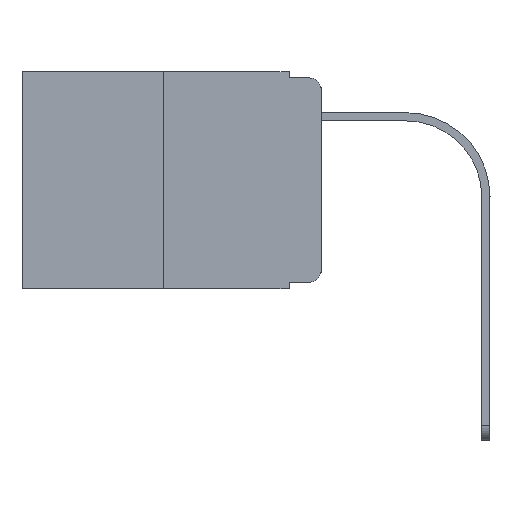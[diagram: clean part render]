
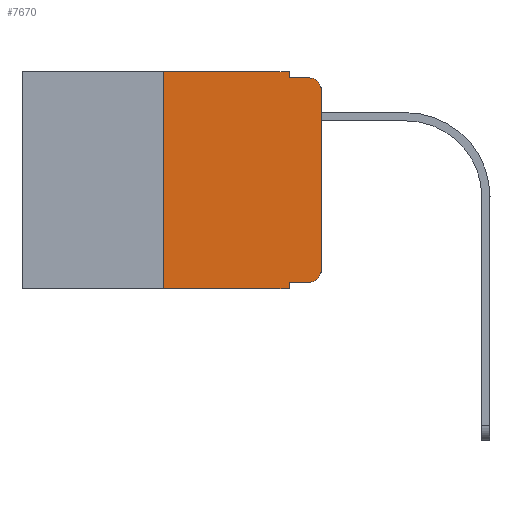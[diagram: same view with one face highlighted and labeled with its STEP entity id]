
A CAD part, left-side view. The second image highlights one B-rep face of the part: STEP entity #7670.
In plain terms, the highlighted planar face has unit normal (-1, 0, 0).
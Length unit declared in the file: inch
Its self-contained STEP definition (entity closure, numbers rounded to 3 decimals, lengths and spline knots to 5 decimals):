
#72 = ORIENTED_EDGE ( 'NONE', *, *, #3887, .T. ) ;
#78 = DIRECTION ( 'NONE',  ( -1., 0., 0. ) ) ;
#151 = CARTESIAN_POINT ( 'NONE',  ( 0., 0.473, 0. ) ) ;
#175 = VERTEX_POINT ( 'NONE', #3811 ) ;
#650 = CARTESIAN_POINT ( 'NONE',  ( 0., 0.25, 0. ) ) ;
#834 = FACE_OUTER_BOUND ( 'NONE', #10438, .T. ) ;
#1130 = VECTOR ( 'NONE', #8430, 39.37008 ) ;
#1160 = DIRECTION ( 'NONE',  ( 0., 0., -1. ) ) ;
#1174 = LINE ( 'NONE', #5401, #1667 ) ;
#1454 = VERTEX_POINT ( 'NONE', #7032 ) ;
#1511 = LINE ( 'NONE', #5705, #4065 ) ;
#1522 = EDGE_CURVE ( 'NONE', #1454, #3395, #8868, .T. ) ;
#1667 = VECTOR ( 'NONE', #9541, 39.37008 ) ;
#1795 = DIRECTION ( 'NONE',  ( 0., -1., 0. ) ) ;
#1896 = DIRECTION ( 'NONE',  ( 1., 0., 0. ) ) ;
#1957 = LINE ( 'NONE', #151, #4524 ) ;
#2030 = VERTEX_POINT ( 'NONE', #5943 ) ;
#2083 = CARTESIAN_POINT ( 'NONE',  ( 0., 0.051, -0.333 ) ) ;
#2164 = CARTESIAN_POINT ( 'NONE',  ( 0., 0., 0. ) ) ;
#2345 = CARTESIAN_POINT ( 'NONE',  ( 0., 0., -0.313 ) ) ;
#2362 = VERTEX_POINT ( 'NONE', #10074 ) ;
#2467 = EDGE_CURVE ( 'NONE', #8702, #10439, #1957, .T. ) ;
#2486 = CARTESIAN_POINT ( 'NONE',  ( 0., 0.051, 0. ) ) ;
#2540 = EDGE_CURVE ( 'NONE', #6546, #175, #1174, .T. ) ;
#2632 = LINE ( 'NONE', #6116, #4465 ) ;
#2684 = DIRECTION ( 'NONE',  ( 0., 0., -1. ) ) ;
#2714 = CARTESIAN_POINT ( 'NONE',  ( 0., 0., -0.03 ) ) ;
#2738 = EDGE_CURVE ( 'NONE', #3395, #8111, #6498, .T. ) ;
#2785 = EDGE_CURVE ( 'NONE', #6546, #8702, #4998, .T. ) ;
#2924 = LINE ( 'NONE', #2083, #3303 ) ;
#3303 = VECTOR ( 'NONE', #3873, 39.37008 ) ;
#3395 = VERTEX_POINT ( 'NONE', #2345 ) ;
#3497 = DIRECTION ( 'NONE',  ( 0., 0., -1. ) ) ;
#3516 = CIRCLE ( 'NONE', #6076, 0.02 ) ;
#3558 = EDGE_CURVE ( 'NONE', #4216, #175, #2632, .T. ) ;
#3667 = ORIENTED_EDGE ( 'NONE', *, *, #3558, .F. ) ;
#3811 = CARTESIAN_POINT ( 'NONE',  ( 0., 0.051, -0.343 ) ) ;
#3873 = DIRECTION ( 'NONE',  ( 0., -1., 0. ) ) ;
#3887 = EDGE_CURVE ( 'NONE', #8111, #2030, #3516, .T. ) ;
#3959 = ORIENTED_EDGE ( 'NONE', *, *, #7503, .F. ) ;
#4065 = VECTOR ( 'NONE', #9330, 39.37008 ) ;
#4216 = VERTEX_POINT ( 'NONE', #8307 ) ;
#4282 = EDGE_CURVE ( 'NONE', #10439, #2362, #8587, .T. ) ;
#4465 = VECTOR ( 'NONE', #2684, 39.37008 ) ;
#4524 = VECTOR ( 'NONE', #1795, 39.37008 ) ;
#4706 = DIRECTION ( 'NONE',  ( 0., 0., -1. ) ) ;
#4998 = LINE ( 'NONE', #650, #1130 ) ;
#5224 = PLANE ( 'NONE',  #8752 ) ;
#5381 = CARTESIAN_POINT ( 'NONE',  ( 0., 0.02, -0.313 ) ) ;
#5401 = CARTESIAN_POINT ( 'NONE',  ( 0., 0.473, -0.343 ) ) ;
#5634 = DIRECTION ( 'NONE',  ( 0., 0., 1. ) ) ;
#5705 = CARTESIAN_POINT ( 'NONE',  ( 0., 0.051, -0.01 ) ) ;
#5925 = CARTESIAN_POINT ( 'NONE',  ( 0., 0.051, 0. ) ) ;
#5943 = CARTESIAN_POINT ( 'NONE',  ( 0., 0.02, -0.01 ) ) ;
#6076 = AXIS2_PLACEMENT_3D ( 'NONE', #7713, #78, #7817 ) ;
#6102 = CARTESIAN_POINT ( 'NONE',  ( 0., 0.25, -0.343 ) ) ;
#6116 = CARTESIAN_POINT ( 'NONE',  ( 0., 0.051, 0. ) ) ;
#6498 = LINE ( 'NONE', #2164, #7420 ) ;
#6546 = VERTEX_POINT ( 'NONE', #6102 ) ;
#7032 = CARTESIAN_POINT ( 'NONE',  ( 0., 0.02, -0.333 ) ) ;
#7420 = VECTOR ( 'NONE', #5634, 39.37008 ) ;
#7503 = EDGE_CURVE ( 'NONE', #2362, #2030, #1511, .T. ) ;
#7670 = ADVANCED_FACE ( 'NONE', ( #834 ), #5224, .F. ) ;
#7699 = VECTOR ( 'NONE', #3497, 39.37008 ) ;
#7713 = CARTESIAN_POINT ( 'NONE',  ( 0., 0.02, -0.03 ) ) ;
#7721 = CARTESIAN_POINT ( 'NONE',  ( 0., 0.473, 0. ) ) ;
#7817 = DIRECTION ( 'NONE',  ( 0., 0., -1. ) ) ;
#8111 = VERTEX_POINT ( 'NONE', #2714 ) ;
#8307 = CARTESIAN_POINT ( 'NONE',  ( 0., 0.051, -0.333 ) ) ;
#8339 = ORIENTED_EDGE ( 'NONE', *, *, #2738, .T. ) ;
#8430 = DIRECTION ( 'NONE',  ( 0., 0., 1. ) ) ;
#8587 = LINE ( 'NONE', #2486, #7699 ) ;
#8623 = ORIENTED_EDGE ( 'NONE', *, *, #4282, .F. ) ;
#8692 = AXIS2_PLACEMENT_3D ( 'NONE', #5381, #8928, #1160 ) ;
#8702 = VERTEX_POINT ( 'NONE', #9436 ) ;
#8752 = AXIS2_PLACEMENT_3D ( 'NONE', #7721, #1896, #4706 ) ;
#8826 = ORIENTED_EDGE ( 'NONE', *, *, #2467, .F. ) ;
#8828 = ORIENTED_EDGE ( 'NONE', *, *, #11093, .T. ) ;
#8868 = CIRCLE ( 'NONE', #8692, 0.02 ) ;
#8928 = DIRECTION ( 'NONE',  ( -1., 0., 0. ) ) ;
#8986 = ORIENTED_EDGE ( 'NONE', *, *, #1522, .T. ) ;
#9330 = DIRECTION ( 'NONE',  ( 0., -1., 0. ) ) ;
#9436 = CARTESIAN_POINT ( 'NONE',  ( 0., 0.25, 0. ) ) ;
#9541 = DIRECTION ( 'NONE',  ( 0., -1., 0. ) ) ;
#9799 = ORIENTED_EDGE ( 'NONE', *, *, #2785, .F. ) ;
#10074 = CARTESIAN_POINT ( 'NONE',  ( 0., 0.051, -0.01 ) ) ;
#10136 = ORIENTED_EDGE ( 'NONE', *, *, #2540, .T. ) ;
#10438 = EDGE_LOOP ( 'NONE', ( #8339, #72, #3959, #8623, #8826, #9799, #10136, #3667, #8828, #8986 ) ) ;
#10439 = VERTEX_POINT ( 'NONE', #5925 ) ;
#11093 = EDGE_CURVE ( 'NONE', #4216, #1454, #2924, .T. ) ;
